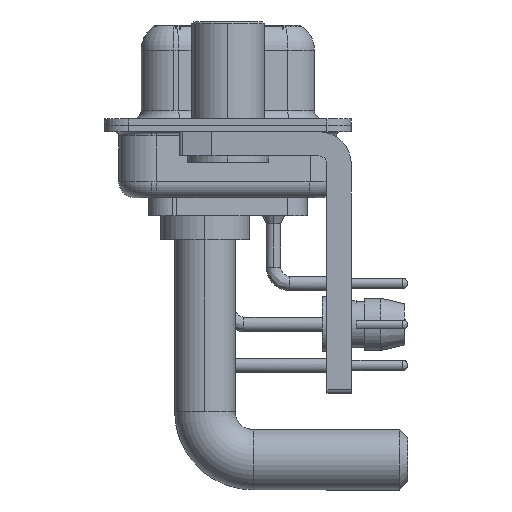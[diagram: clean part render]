
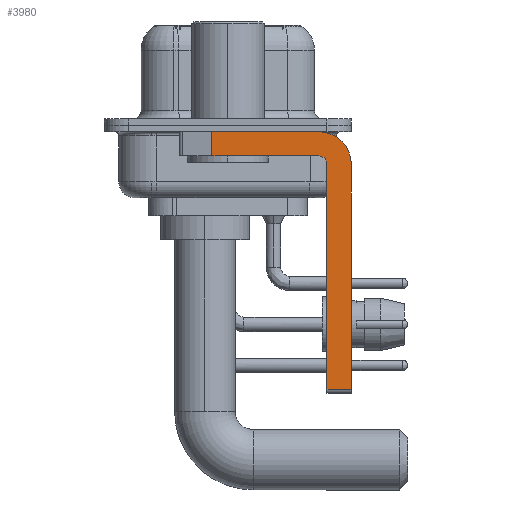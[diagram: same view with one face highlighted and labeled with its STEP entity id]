
A CAD part, left-side view. The second image highlights one B-rep face of the part: STEP entity #3980.
In plain terms, the highlighted planar face has unit normal (-1, 0, 0).
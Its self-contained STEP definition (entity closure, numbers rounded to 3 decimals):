
#50 = DIRECTION ( 'NONE',  ( 0., -1., 0. ) ) ;
#695 = CARTESIAN_POINT ( 'NONE',  ( -2.9, -6.15, -16.6 ) ) ;
#1273 = EDGE_CURVE ( 'NONE', #18025, #12642, #32593, .T. ) ;
#1308 = FACE_OUTER_BOUND ( 'NONE', #13922, .T. ) ;
#1599 = CARTESIAN_POINT ( 'NONE',  ( -2.9, -6.15, -2.4 ) ) ;
#2217 = CARTESIAN_POINT ( 'NONE',  ( -2.9, -7.65, -2.4 ) ) ;
#2820 = CARTESIAN_POINT ( 'NONE',  ( -2.9, 3., -0.4 ) ) ;
#3207 = VECTOR ( 'NONE', #50, 1000. ) ;
#3980 = ADVANCED_FACE ( 'NONE', ( #1308 ), #18918, .F. ) ;
#5578 = CARTESIAN_POINT ( 'NONE',  ( -2.9, 0.978, -0.4 ) ) ;
#5906 = VERTEX_POINT ( 'NONE', #19060 ) ;
#5957 = LINE ( 'NONE', #2820, #3207 ) ;
#6605 = DIRECTION ( 'NONE',  ( 0., 0., 1. ) ) ;
#6684 = VECTOR ( 'NONE', #9167, 1000. ) ;
#7388 = CARTESIAN_POINT ( 'NONE',  ( -2.9, -5.65, -2.4 ) ) ;
#7574 = EDGE_CURVE ( 'NONE', #20842, #16862, #33507, .T. ) ;
#7729 = DIRECTION ( 'NONE',  ( 1., 0., 0. ) ) ;
#7751 = CARTESIAN_POINT ( 'NONE',  ( -2.9, 0.978, -1.9 ) ) ;
#8543 = VERTEX_POINT ( 'NONE', #12994 ) ;
#8898 = VERTEX_POINT ( 'NONE', #5578 ) ;
#9167 = DIRECTION ( 'NONE',  ( 0., 0., -1. ) ) ;
#9235 = ORIENTED_EDGE ( 'NONE', *, *, #1273, .F. ) ;
#9961 = AXIS2_PLACEMENT_3D ( 'NONE', #13291, #7729, #12932 ) ;
#10274 = CARTESIAN_POINT ( 'NONE',  ( -2.9, -5.65, -1.9 ) ) ;
#10663 = CARTESIAN_POINT ( 'NONE',  ( -2.9, -5.65, -1.9 ) ) ;
#10868 = LINE ( 'NONE', #21811, #23362 ) ;
#11035 = DIRECTION ( 'NONE',  ( 0., 1., 0. ) ) ;
#11119 = AXIS2_PLACEMENT_3D ( 'NONE', #25406, #14081, #30973 ) ;
#11166 = CIRCLE ( 'NONE', #9961, 2. ) ;
#12597 = EDGE_CURVE ( 'NONE', #13850, #8543, #16677, .T. ) ;
#12642 = VERTEX_POINT ( 'NONE', #1599 ) ;
#12932 = DIRECTION ( 'NONE',  ( 0., 0., -1. ) ) ;
#12994 = CARTESIAN_POINT ( 'NONE',  ( -2.9, -7.65, -16.35 ) ) ;
#13291 = CARTESIAN_POINT ( 'NONE',  ( -2.9, -5.65, -2.4 ) ) ;
#13480 = EDGE_CURVE ( 'NONE', #8898, #5906, #5957, .T. ) ;
#13850 = VERTEX_POINT ( 'NONE', #20158 ) ;
#13922 = EDGE_LOOP ( 'NONE', ( #34070, #26233, #35870, #32498, #9235, #15529, #34381, #24055 ) ) ;
#14081 = DIRECTION ( 'NONE',  ( -1., 0., 0. ) ) ;
#15529 = ORIENTED_EDGE ( 'NONE', *, *, #19857, .T. ) ;
#16673 = LINE ( 'NONE', #25006, #31672 ) ;
#16677 = LINE ( 'NONE', #2217, #6684 ) ;
#16862 = VERTEX_POINT ( 'NONE', #7751 ) ;
#18025 = VERTEX_POINT ( 'NONE', #22248 ) ;
#18359 = DIRECTION ( 'NONE',  ( 0., 0., -1. ) ) ;
#18918 = PLANE ( 'NONE',  #32631 ) ;
#19060 = CARTESIAN_POINT ( 'NONE',  ( -2.9, -5.65, -0.4 ) ) ;
#19857 = EDGE_CURVE ( 'NONE', #18025, #8543, #16673, .T. ) ;
#20158 = CARTESIAN_POINT ( 'NONE',  ( -2.9, -7.65, -2.4 ) ) ;
#20192 = EDGE_CURVE ( 'NONE', #8898, #16862, #10868, .T. ) ;
#20433 = VECTOR ( 'NONE', #6605, 1000. ) ;
#20842 = VERTEX_POINT ( 'NONE', #10274 ) ;
#21811 = CARTESIAN_POINT ( 'NONE',  ( -2.9, 0.978, -1.9 ) ) ;
#22037 = DIRECTION ( 'NONE',  ( 0., -1., 0. ) ) ;
#22248 = CARTESIAN_POINT ( 'NONE',  ( -2.9, -6.15, -16.35 ) ) ;
#23362 = VECTOR ( 'NONE', #27953, 1000. ) ;
#24055 = ORIENTED_EDGE ( 'NONE', *, *, #34953, .F. ) ;
#24515 = EDGE_CURVE ( 'NONE', #12642, #20842, #33068, .T. ) ;
#25006 = CARTESIAN_POINT ( 'NONE',  ( -2.9, -5.65, -16.35 ) ) ;
#25406 = CARTESIAN_POINT ( 'NONE',  ( -2.9, -5.65, -2.4 ) ) ;
#26233 = ORIENTED_EDGE ( 'NONE', *, *, #20192, .T. ) ;
#27953 = DIRECTION ( 'NONE',  ( 0., 0., -1. ) ) ;
#29679 = DIRECTION ( 'NONE',  ( 1., 0., 0. ) ) ;
#30973 = DIRECTION ( 'NONE',  ( 0., 0., 1. ) ) ;
#31672 = VECTOR ( 'NONE', #22037, 1000. ) ;
#32498 = ORIENTED_EDGE ( 'NONE', *, *, #24515, .F. ) ;
#32593 = LINE ( 'NONE', #695, #20433 ) ;
#32631 = AXIS2_PLACEMENT_3D ( 'NONE', #7388, #29679, #18359 ) ;
#33068 = CIRCLE ( 'NONE', #11119, 0.5 ) ;
#33507 = LINE ( 'NONE', #10663, #35504 ) ;
#34070 = ORIENTED_EDGE ( 'NONE', *, *, #13480, .F. ) ;
#34381 = ORIENTED_EDGE ( 'NONE', *, *, #12597, .F. ) ;
#34953 = EDGE_CURVE ( 'NONE', #5906, #13850, #11166, .T. ) ;
#35504 = VECTOR ( 'NONE', #11035, 1000. ) ;
#35870 = ORIENTED_EDGE ( 'NONE', *, *, #7574, .F. ) ;
